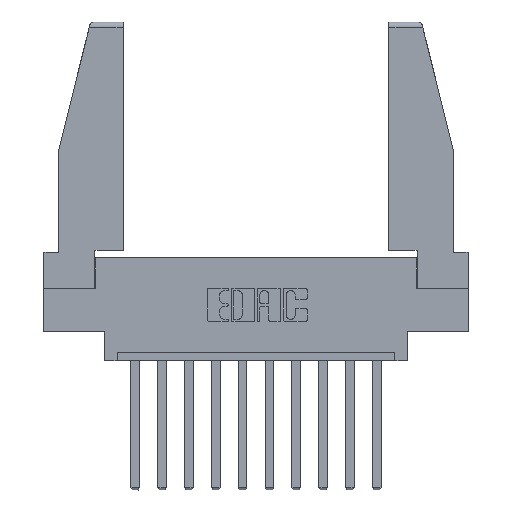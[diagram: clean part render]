
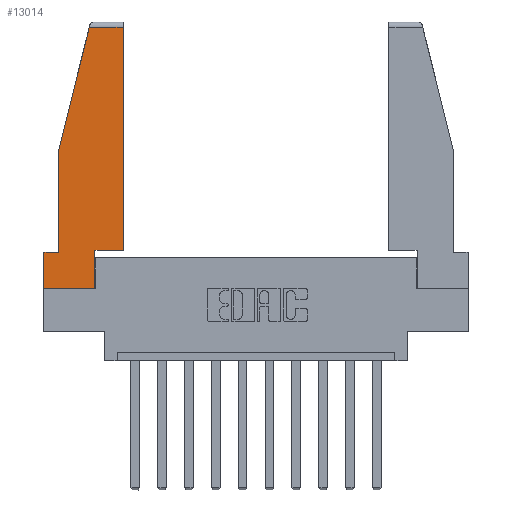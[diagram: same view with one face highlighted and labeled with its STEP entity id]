
A CAD part, top view. The second image highlights one B-rep face of the part: STEP entity #13014.
In plain terms, the highlighted planar face has unit normal (0, 0, 1).
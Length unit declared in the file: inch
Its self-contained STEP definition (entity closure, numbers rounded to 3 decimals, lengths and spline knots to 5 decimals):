
#78 = LINE ( 'NONE', #7092, #12040 ) ;
#286 = ORIENTED_EDGE ( 'NONE', *, *, #13897, .T. ) ;
#320 = CARTESIAN_POINT ( 'NONE',  ( 0.2636, 1.52, 0. ) ) ;
#485 = VERTEX_POINT ( 'NONE', #5765 ) ;
#552 = DIRECTION ( 'NONE',  ( 1., 0., 0. ) ) ;
#566 = LINE ( 'NONE', #11730, #13910 ) ;
#1117 = ORIENTED_EDGE ( 'NONE', *, *, #7962, .T. ) ;
#1478 = EDGE_LOOP ( 'NONE', ( #1117, #2498, #12575, #11384, #7900, #286, #10728, #11946, #11661 ) ) ;
#1671 = EDGE_CURVE ( 'NONE', #2337, #9583, #2380, .T. ) ;
#2221 = CARTESIAN_POINT ( 'NONE',  ( 0., 0., 0. ) ) ;
#2337 = VERTEX_POINT ( 'NONE', #10235 ) ;
#2380 = LINE ( 'NONE', #13580, #4429 ) ;
#2475 = VECTOR ( 'NONE', #8260, 39.37008 ) ;
#2498 = ORIENTED_EDGE ( 'NONE', *, *, #4607, .T. ) ;
#2650 = VERTEX_POINT ( 'NONE', #9347 ) ;
#2707 = VERTEX_POINT ( 'NONE', #13725 ) ;
#2788 = EDGE_CURVE ( 'NONE', #2707, #10081, #13495, .T. ) ;
#2975 = EDGE_CURVE ( 'NONE', #2650, #3368, #4055, .T. ) ;
#2984 = CARTESIAN_POINT ( 'NONE',  ( 0., 0.21, 0. ) ) ;
#3366 = DIRECTION ( 'NONE',  ( 1., 0., 0. ) ) ;
#3368 = VERTEX_POINT ( 'NONE', #11967 ) ;
#3690 = CARTESIAN_POINT ( 'NONE',  ( 0., 1.52, 0. ) ) ;
#3773 = PLANE ( 'NONE',  #8289 ) ;
#3878 = DIRECTION ( 'NONE',  ( 0., -1., 0. ) ) ;
#3969 = VECTOR ( 'NONE', #10812, 39.37008 ) ;
#4055 = LINE ( 'NONE', #2221, #12463 ) ;
#4429 = VECTOR ( 'NONE', #3878, 39.37008 ) ;
#4607 = EDGE_CURVE ( 'NONE', #485, #6190, #9575, .T. ) ;
#4869 = DIRECTION ( 'NONE',  ( 0., 0., 1. ) ) ;
#5048 = DIRECTION ( 'NONE',  ( 0., -1., 0. ) ) ;
#5765 = CARTESIAN_POINT ( 'NONE',  ( 0.461, 1.52, 0. ) ) ;
#5865 = VECTOR ( 'NONE', #6759, 39.37008 ) ;
#6190 = VERTEX_POINT ( 'NONE', #320 ) ;
#6338 = EDGE_CURVE ( 'NONE', #6190, #2337, #10109, .T. ) ;
#6759 = DIRECTION ( 'NONE',  ( -1., 0., 0. ) ) ;
#7092 = CARTESIAN_POINT ( 'NONE',  ( 0., 0.21, 0. ) ) ;
#7778 = CARTESIAN_POINT ( 'NONE',  ( 0.086, 0.21, 0. ) ) ;
#7900 = ORIENTED_EDGE ( 'NONE', *, *, #10386, .T. ) ;
#7962 = EDGE_CURVE ( 'NONE', #10081, #485, #13113, .T. ) ;
#8041 = CARTESIAN_POINT ( 'NONE',  ( 0.297, 0.223, 0. ) ) ;
#8260 = DIRECTION ( 'NONE',  ( 0., 1., 0. ) ) ;
#8289 = AXIS2_PLACEMENT_3D ( 'NONE', #13430, #4869, #552 ) ;
#9347 = CARTESIAN_POINT ( 'NONE',  ( 0., 0., 0. ) ) ;
#9452 = VERTEX_POINT ( 'NONE', #2984 ) ;
#9575 = LINE ( 'NONE', #3690, #5865 ) ;
#9583 = VERTEX_POINT ( 'NONE', #7778 ) ;
#9785 = CARTESIAN_POINT ( 'NONE',  ( 0.297, 0., 0. ) ) ;
#10081 = VERTEX_POINT ( 'NONE', #13296 ) ;
#10109 = LINE ( 'NONE', #11909, #12659 ) ;
#10235 = CARTESIAN_POINT ( 'NONE',  ( 0.086, 0.8, 0. ) ) ;
#10386 = EDGE_CURVE ( 'NONE', #9583, #9452, #566, .T. ) ;
#10543 = CARTESIAN_POINT ( 'NONE',  ( 0.461, 0.223, 0. ) ) ;
#10728 = ORIENTED_EDGE ( 'NONE', *, *, #2975, .T. ) ;
#10812 = DIRECTION ( 'NONE',  ( 0., 1., 0. ) ) ;
#11384 = ORIENTED_EDGE ( 'NONE', *, *, #1671, .T. ) ;
#11408 = DIRECTION ( 'NONE',  ( 1., 0., 0. ) ) ;
#11612 = VECTOR ( 'NONE', #11408, 39.37008 ) ;
#11661 = ORIENTED_EDGE ( 'NONE', *, *, #2788, .T. ) ;
#11674 = DIRECTION ( 'NONE',  ( -1., 0., 0. ) ) ;
#11730 = CARTESIAN_POINT ( 'NONE',  ( 0., 0.21, 0. ) ) ;
#11785 = EDGE_CURVE ( 'NONE', #3368, #2707, #13055, .T. ) ;
#11909 = CARTESIAN_POINT ( 'NONE',  ( 0.271, 1.55, 0. ) ) ;
#11946 = ORIENTED_EDGE ( 'NONE', *, *, #11785, .T. ) ;
#11967 = CARTESIAN_POINT ( 'NONE',  ( 0.297, 0., 0. ) ) ;
#12040 = VECTOR ( 'NONE', #5048, 39.37008 ) ;
#12184 = DIRECTION ( 'NONE',  ( -0.239, -0.971, 0. ) ) ;
#12463 = VECTOR ( 'NONE', #3366, 39.37008 ) ;
#12575 = ORIENTED_EDGE ( 'NONE', *, *, #6338, .T. ) ;
#12659 = VECTOR ( 'NONE', #12184, 39.37008 ) ;
#13014 = ADVANCED_FACE ( 'NONE', ( #13015 ), #3773, .T. ) ;
#13015 = FACE_OUTER_BOUND ( 'NONE', #1478, .T. ) ;
#13055 = LINE ( 'NONE', #9785, #3969 ) ;
#13113 = LINE ( 'NONE', #10543, #2475 ) ;
#13296 = CARTESIAN_POINT ( 'NONE',  ( 0.461, 0.223, 0. ) ) ;
#13430 = CARTESIAN_POINT ( 'NONE',  ( 0., 0., 0. ) ) ;
#13495 = LINE ( 'NONE', #8041, #11612 ) ;
#13580 = CARTESIAN_POINT ( 'NONE',  ( 0.086, 0.8, 0. ) ) ;
#13725 = CARTESIAN_POINT ( 'NONE',  ( 0.297, 0.223, 0. ) ) ;
#13897 = EDGE_CURVE ( 'NONE', #9452, #2650, #78, .T. ) ;
#13910 = VECTOR ( 'NONE', #11674, 39.37008 ) ;
